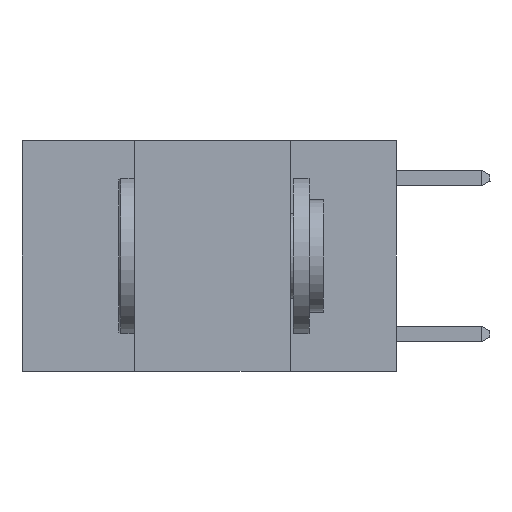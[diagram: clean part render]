
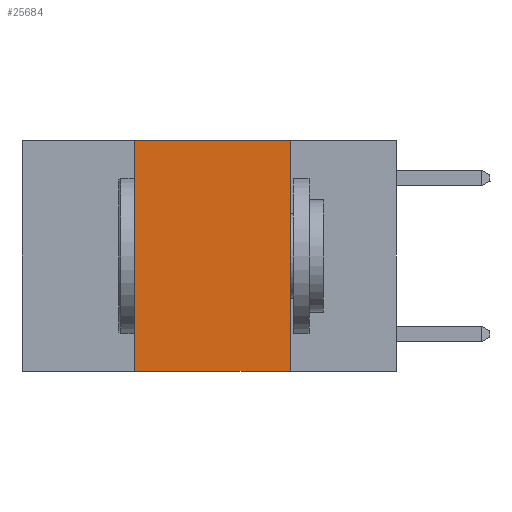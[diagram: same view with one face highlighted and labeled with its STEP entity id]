
A CAD part, left-side view. The second image highlights one B-rep face of the part: STEP entity #25684.
In plain terms, the highlighted planar face has unit normal (-1, 0, 0).
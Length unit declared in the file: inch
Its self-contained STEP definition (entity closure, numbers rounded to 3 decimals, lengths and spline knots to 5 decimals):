
#1256 = CARTESIAN_POINT ( 'NONE',  ( 0., 0.6, 0. ) ) ;
#1328 = DIRECTION ( 'NONE',  ( 0., -1., 0. ) ) ;
#3719 = VERTEX_POINT ( 'NONE', #10566 ) ;
#4233 = LINE ( 'NONE', #13056, #16494 ) ;
#5993 = VECTOR ( 'NONE', #1328, 39.37008 ) ;
#6672 = CARTESIAN_POINT ( 'NONE',  ( 0., 0.17, -0.37 ) ) ;
#6824 = PLANE ( 'NONE',  #10159 ) ;
#9150 = DIRECTION ( 'NONE',  ( 0., 0., -1. ) ) ;
#9688 = FACE_OUTER_BOUND ( 'NONE', #13025, .T. ) ;
#10159 = AXIS2_PLACEMENT_3D ( 'NONE', #16011, #22948, #9150 ) ;
#10566 = CARTESIAN_POINT ( 'NONE',  ( 0., 0.42, -0.37 ) ) ;
#12781 = VECTOR ( 'NONE', #17233, 39.37008 ) ;
#13025 = EDGE_LOOP ( 'NONE', ( #17008, #13581, #14522, #15998 ) ) ;
#13056 = CARTESIAN_POINT ( 'NONE',  ( 0., 0.17, 0. ) ) ;
#13378 = CARTESIAN_POINT ( 'NONE',  ( 0., 0.42, 0. ) ) ;
#13581 = ORIENTED_EDGE ( 'NONE', *, *, #20072, .F. ) ;
#14196 = VERTEX_POINT ( 'NONE', #6672 ) ;
#14242 = LINE ( 'NONE', #21835, #12781 ) ;
#14522 = ORIENTED_EDGE ( 'NONE', *, *, #28410, .F. ) ;
#15351 = DIRECTION ( 'NONE',  ( 0., 0., -1. ) ) ;
#15746 = CARTESIAN_POINT ( 'NONE',  ( 0., 0.17, 0. ) ) ;
#15998 = ORIENTED_EDGE ( 'NONE', *, *, #18750, .T. ) ;
#16011 = CARTESIAN_POINT ( 'NONE',  ( 0., 0.6, 0. ) ) ;
#16494 = VECTOR ( 'NONE', #15351, 39.37008 ) ;
#17008 = ORIENTED_EDGE ( 'NONE', *, *, #17663, .F. ) ;
#17233 = DIRECTION ( 'NONE',  ( 0., 0., 1. ) ) ;
#17320 = DIRECTION ( 'NONE',  ( 0., -1., 0. ) ) ;
#17663 = EDGE_CURVE ( 'NONE', #18900, #14196, #4233, .T. ) ;
#18750 = EDGE_CURVE ( 'NONE', #3719, #14196, #18964, .T. ) ;
#18864 = VERTEX_POINT ( 'NONE', #13378 ) ;
#18900 = VERTEX_POINT ( 'NONE', #15746 ) ;
#18964 = LINE ( 'NONE', #28582, #5993 ) ;
#20072 = EDGE_CURVE ( 'NONE', #18864, #18900, #24229, .T. ) ;
#21835 = CARTESIAN_POINT ( 'NONE',  ( 0., 0.42, 0. ) ) ;
#22948 = DIRECTION ( 'NONE',  ( 1., 0., 0. ) ) ;
#24229 = LINE ( 'NONE', #1256, #24908 ) ;
#24908 = VECTOR ( 'NONE', #17320, 39.37008 ) ;
#25684 = ADVANCED_FACE ( 'NONE', ( #9688 ), #6824, .F. ) ;
#28410 = EDGE_CURVE ( 'NONE', #3719, #18864, #14242, .T. ) ;
#28582 = CARTESIAN_POINT ( 'NONE',  ( 0., 0.6, -0.37 ) ) ;
